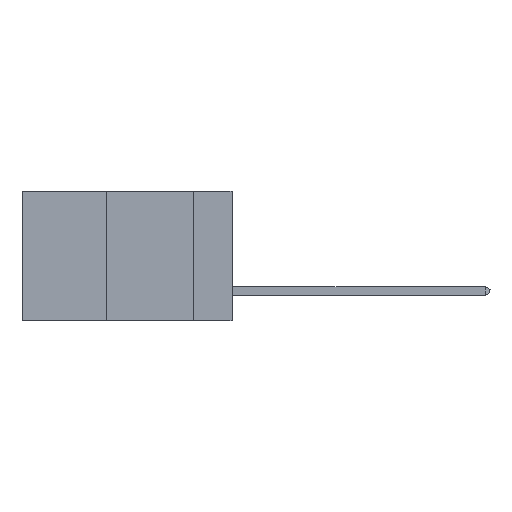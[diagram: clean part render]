
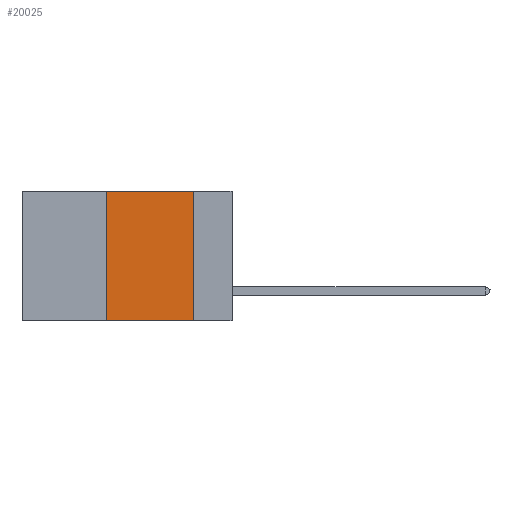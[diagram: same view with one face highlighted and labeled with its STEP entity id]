
A CAD part, left-side view. The second image highlights one B-rep face of the part: STEP entity #20025.
In plain terms, the highlighted planar face has unit normal (-1, 0, 0).
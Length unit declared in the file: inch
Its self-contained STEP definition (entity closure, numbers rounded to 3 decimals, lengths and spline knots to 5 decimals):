
#1795 = VECTOR ( 'NONE', #30539, 39.37008 ) ;
#2306 = EDGE_CURVE ( 'NONE', #22143, #30032, #14755, .T. ) ;
#3622 = FACE_OUTER_BOUND ( 'NONE', #11864, .T. ) ;
#3952 = ORIENTED_EDGE ( 'NONE', *, *, #11911, .T. ) ;
#4938 = CARTESIAN_POINT ( 'NONE',  ( 0., 0.6, 0. ) ) ;
#5376 = EDGE_CURVE ( 'NONE', #17972, #22143, #22552, .T. ) ;
#5835 = CARTESIAN_POINT ( 'NONE',  ( 0., 0.11, 0. ) ) ;
#8785 = DIRECTION ( 'NONE',  ( 0., 0., -1. ) ) ;
#8800 = LINE ( 'NONE', #10705, #1795 ) ;
#8915 = CARTESIAN_POINT ( 'NONE',  ( 0., 0.11, 0. ) ) ;
#10705 = CARTESIAN_POINT ( 'NONE',  ( 0., 0.6, -0.37 ) ) ;
#10952 = DIRECTION ( 'NONE',  ( 0., 0., -1. ) ) ;
#11262 = DIRECTION ( 'NONE',  ( 1., 0., 0. ) ) ;
#11864 = EDGE_LOOP ( 'NONE', ( #16537, #18774, #13141, #3952 ) ) ;
#11911 = EDGE_CURVE ( 'NONE', #27543, #30032, #8800, .T. ) ;
#13087 = CARTESIAN_POINT ( 'NONE',  ( 0., 0.36, -0.37 ) ) ;
#13141 = ORIENTED_EDGE ( 'NONE', *, *, #20187, .F. ) ;
#13986 = CARTESIAN_POINT ( 'NONE',  ( 0., 0.11, -0.37 ) ) ;
#14506 = DIRECTION ( 'NONE',  ( 0., 0., 1. ) ) ;
#14755 = LINE ( 'NONE', #5835, #16658 ) ;
#16050 = LINE ( 'NONE', #19347, #23403 ) ;
#16537 = ORIENTED_EDGE ( 'NONE', *, *, #2306, .F. ) ;
#16658 = VECTOR ( 'NONE', #10952, 39.37008 ) ;
#17972 = VERTEX_POINT ( 'NONE', #26958 ) ;
#18774 = ORIENTED_EDGE ( 'NONE', *, *, #5376, .F. ) ;
#19347 = CARTESIAN_POINT ( 'NONE',  ( 0., 0.36, 0. ) ) ;
#20025 = ADVANCED_FACE ( 'NONE', ( #3622 ), #25347, .F. ) ;
#20187 = EDGE_CURVE ( 'NONE', #27543, #17972, #16050, .T. ) ;
#20601 = VECTOR ( 'NONE', #27278, 39.37008 ) ;
#22143 = VERTEX_POINT ( 'NONE', #8915 ) ;
#22552 = LINE ( 'NONE', #4938, #20601 ) ;
#23403 = VECTOR ( 'NONE', #14506, 39.37008 ) ;
#23604 = CARTESIAN_POINT ( 'NONE',  ( 0., 0.6, 0. ) ) ;
#24641 = AXIS2_PLACEMENT_3D ( 'NONE', #23604, #11262, #8785 ) ;
#25347 = PLANE ( 'NONE',  #24641 ) ;
#26958 = CARTESIAN_POINT ( 'NONE',  ( 0., 0.36, 0. ) ) ;
#27278 = DIRECTION ( 'NONE',  ( 0., -1., 0. ) ) ;
#27543 = VERTEX_POINT ( 'NONE', #13087 ) ;
#30032 = VERTEX_POINT ( 'NONE', #13986 ) ;
#30539 = DIRECTION ( 'NONE',  ( 0., -1., 0. ) ) ;
